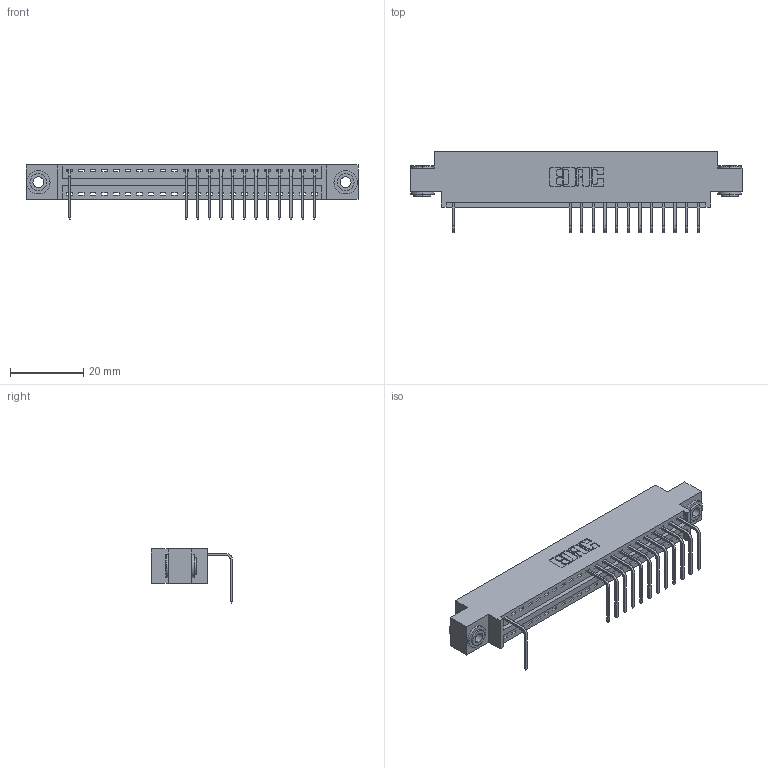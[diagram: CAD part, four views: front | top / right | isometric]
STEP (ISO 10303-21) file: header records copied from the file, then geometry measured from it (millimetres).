
FILE_DESCRIPTION (( 'STEP AP203' ), '1' );
FILE_NAME ('346-022-558-603.STEP', '2018-08-21T01:08:29', ( '' ), ( '' ), 'SwSTEP 2.0', 'SolidWorks 2016', '' );
FILE_SCHEMA (( 'CONFIG_CONTROL_DESIGN' ));
Length unit declared in the file: inch
Products named in the file (4): 345-292-001_558 Tail - 2; 345-250-002_345-250-002-102; 346-022-558-603; 346 Part_0.170 Offset - 0.156 Dia-TH
Assembly tree (16 placements, depth 2):
  346-022-558-603
    346 Part_0.170 Offset - 0.156 Dia-TH
    345-292-001_558 Tail - 2  x13
    345-250-002_345-250-002-102  x2
Bounding box: 90.42 x 22.16 x 14.73 mm (x, y, z)
Volume: 8323 mm3; surface area: 10270.9 mm2
Topology: 16 solids, 16 shells, 1052 faces, 3161 edges, 2086 vertices
Faces by surface type: plane 726, cylinder 318, cone 8
Entity records: 16924 total; most frequent: CARTESIAN_POINT 2928, ORIENTED_EDGE 2886, DIRECTION 2627, EDGE_CURVE 1443, VECTOR 1199, LINE 1199, VERTEX_POINT 958, AXIS2_PLACEMENT_3D 714
